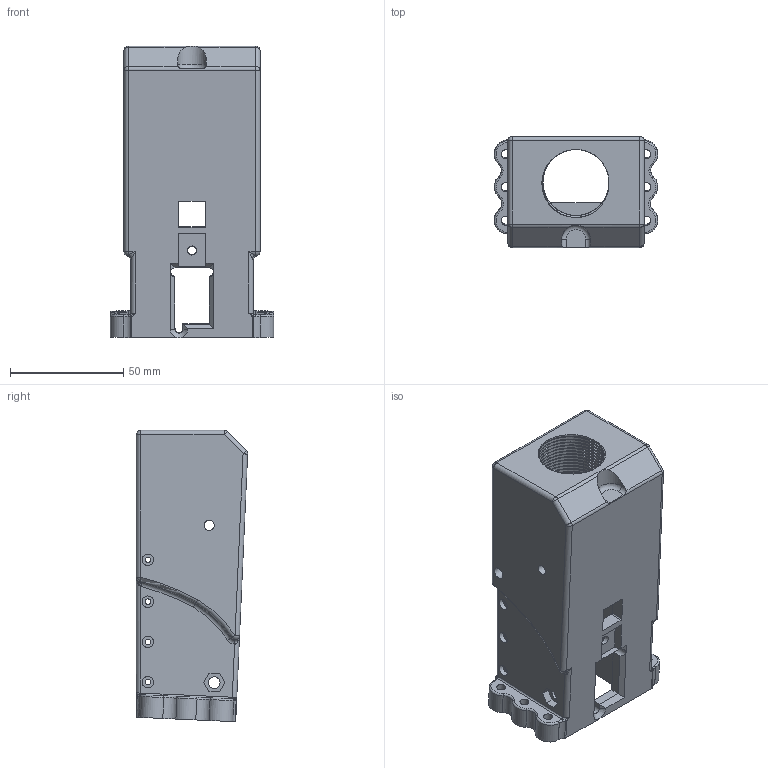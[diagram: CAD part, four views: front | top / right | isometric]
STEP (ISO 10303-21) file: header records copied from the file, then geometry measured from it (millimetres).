
FILE_DESCRIPTION(/* description */ (''),/* implementation_level */ '2;1');
FILE_NAME(/* name */ 'Plastikov v2.1 Rear Receiver AR15 Stock.stp',/* time_stamp */ '2020-08-09T23:12:00-05:00',/* author */ ('johne'),/* organization */ (''),/* preprocessor_version */ 'ST-DEVELOPER v18',/* originating_system */ 'Autodesk Inventor 2020',/* authorisation */ '');
FILE_SCHEMA (('AUTOMOTIVE_DESIGN { 1 0 10303 214 3 1 1 }'));
Products named in the file (1): Plastikov v2.0 Rear Receiver AR15 Stock
Bounding box: 72.2 x 49.14 x 128.76 mm (x, y, z)
Volume: 193842.1 mm3; surface area: 45321.3 mm2
Topology: 1 solids, 1 shells, 296 faces, 794 edges, 505 vertices
Faces by surface type: cylinder 117, plane 77, bspline 62, torus 25, sphere 14, cone 1
Full cylindrical faces by diameter (mm): 2.5 x8, 3.12 x4, 4 x7, 4.5 x2, 5.08 x8, 5.1 x2, 12 x1, 29.21 x16, 30.163 x16
Entity records: 33880 total; most frequent: CARTESIAN_POINT 26746, ORIENTED_EDGE 1572, DIRECTION 1330, EDGE_CURVE 786, AXIS2_PLACEMENT_3D 524, VERTEX_POINT 505, EDGE_LOOP 353, FACE_OUTER_BOUND 296
